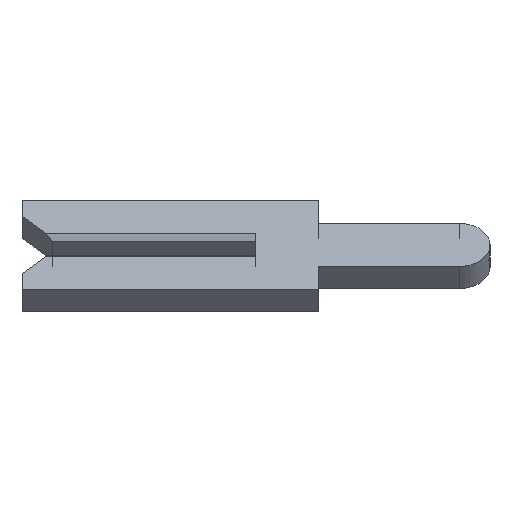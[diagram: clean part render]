
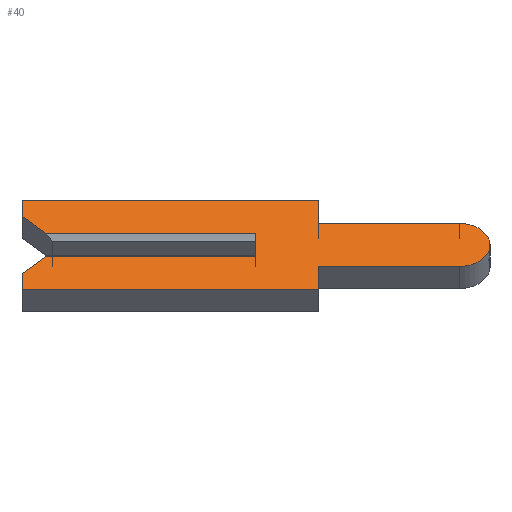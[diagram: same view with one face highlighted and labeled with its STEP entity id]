
A CAD part, left-side view. The second image highlights one B-rep face of the part: STEP entity #40.
In plain terms, the highlighted face is planar.
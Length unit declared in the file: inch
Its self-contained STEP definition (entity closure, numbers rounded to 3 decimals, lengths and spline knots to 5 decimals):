
#7 = CARTESIAN_POINT ( 'NONE',  ( -0.01, -0.1305, -0.0195 ) ) ;
#40 = ADVANCED_FACE ( 'NONE', ( #916 ), #999, .F. ) ;
#54 = CARTESIAN_POINT ( 'NONE',  ( -0.01, 0.15, -0.026 ) ) ;
#56 = ORIENTED_EDGE ( 'NONE', *, *, #1385, .F. ) ;
#73 = VERTEX_POINT ( 'NONE', #1260 ) ;
#75 = ORIENTED_EDGE ( 'NONE', *, *, #737, .T. ) ;
#84 = CARTESIAN_POINT ( 'NONE',  ( -0.01, 0.1305, 0.0065 ) ) ;
#95 = ORIENTED_EDGE ( 'NONE', *, *, #278, .F. ) ;
#117 = EDGE_CURVE ( 'NONE', #73, #673, #1563, .T. ) ;
#166 = VERTEX_POINT ( 'NONE', #751 ) ;
#167 = DIRECTION ( 'NONE',  ( 0., -1., 0. ) ) ;
#184 = VERTEX_POINT ( 'NONE', #244 ) ;
#197 = EDGE_CURVE ( 'NONE', #1098, #594, #1121, .T. ) ;
#206 = EDGE_CURVE ( 'NONE', #1483, #184, #1257, .T. ) ;
#219 = CARTESIAN_POINT ( 'NONE',  ( -0.01, -0.04, 0.0195 ) ) ;
#220 = VECTOR ( 'NONE', #1440, 39.37008 ) ;
#230 = ORIENTED_EDGE ( 'NONE', *, *, #1221, .F. ) ;
#234 = DIRECTION ( 'NONE',  ( 0., -1., 0. ) ) ;
#236 = LINE ( 'NONE', #606, #220 ) ;
#244 = CARTESIAN_POINT ( 'NONE',  ( -0.01, -0.04, -0.0195 ) ) ;
#247 = VECTOR ( 'NONE', #285, 39.37008 ) ;
#265 = EDGE_CURVE ( 'NONE', #673, #735, #1557, .T. ) ;
#269 = CARTESIAN_POINT ( 'NONE',  ( -0.01, 0.15, -0.026 ) ) ;
#278 = EDGE_CURVE ( 'NONE', #1012, #1098, #1266, .T. ) ;
#285 = DIRECTION ( 'NONE',  ( 0., -0.707, 0.707 ) ) ;
#288 = VERTEX_POINT ( 'NONE', #1540 ) ;
#307 = VECTOR ( 'NONE', #618, 39.37008 ) ;
#311 = CARTESIAN_POINT ( 'NONE',  ( -0.01, -0.04, 0.04 ) ) ;
#329 = CARTESIAN_POINT ( 'NONE',  ( -0.01, 0.134, -0.01 ) ) ;
#353 = CARTESIAN_POINT ( 'NONE',  ( -0.01, -0.1305, 0. ) ) ;
#406 = LINE ( 'NONE', #416, #780 ) ;
#416 = CARTESIAN_POINT ( 'NONE',  ( -0.01, 0.15, 0.01 ) ) ;
#423 = EDGE_CURVE ( 'NONE', #735, #1012, #580, .T. ) ;
#460 = LINE ( 'NONE', #1486, #898 ) ;
#465 = ORIENTED_EDGE ( 'NONE', *, *, #1082, .F. ) ;
#471 = DIRECTION ( 'NONE',  ( 1., 0., 0. ) ) ;
#481 = VECTOR ( 'NONE', #234, 39.37008 ) ;
#494 = DIRECTION ( 'NONE',  ( 0., 0., -1. ) ) ;
#540 = ORIENTED_EDGE ( 'NONE', *, *, #1000, .F. ) ;
#569 = AXIS2_PLACEMENT_3D ( 'NONE', #1506, #875, #494 ) ;
#580 = LINE ( 'NONE', #1154, #247 ) ;
#594 = VERTEX_POINT ( 'NONE', #672 ) ;
#598 = DIRECTION ( 'NONE',  ( 0., -1., 0. ) ) ;
#599 = ORIENTED_EDGE ( 'NONE', *, *, #423, .F. ) ;
#605 = LINE ( 'NONE', #940, #802 ) ;
#606 = CARTESIAN_POINT ( 'NONE',  ( -0.01, -0.04, -0.04 ) ) ;
#612 = CARTESIAN_POINT ( 'NONE',  ( -0.01, 0.15, 0.04 ) ) ;
#618 = DIRECTION ( 'NONE',  ( 0., 0., 1. ) ) ;
#635 = ORIENTED_EDGE ( 'NONE', *, *, #265, .F. ) ;
#672 = CARTESIAN_POINT ( 'NONE',  ( -0.01, 0., 0.01 ) ) ;
#673 = VERTEX_POINT ( 'NONE', #815 ) ;
#727 = ORIENTED_EDGE ( 'NONE', *, *, #206, .F. ) ;
#729 = DIRECTION ( 'NONE',  ( 0., 0., -1. ) ) ;
#735 = VERTEX_POINT ( 'NONE', #54 ) ;
#737 = EDGE_CURVE ( 'NONE', #288, #594, #406, .T. ) ;
#744 = VECTOR ( 'NONE', #956, 39.37008 ) ;
#751 = CARTESIAN_POINT ( 'NONE',  ( -0.01, 0.15, 0.04 ) ) ;
#754 = DIRECTION ( 'NONE',  ( 0., 1., 0. ) ) ;
#780 = VECTOR ( 'NONE', #167, 39.37008 ) ;
#802 = VECTOR ( 'NONE', #1096, 39.37008 ) ;
#815 = CARTESIAN_POINT ( 'NONE',  ( -0.01, 0.15, -0.04 ) ) ;
#832 = VERTEX_POINT ( 'NONE', #1432 ) ;
#867 = LINE ( 'NONE', #311, #1512 ) ;
#875 = DIRECTION ( 'NONE',  ( 1., 0., 0. ) ) ;
#886 = DIRECTION ( 'NONE',  ( 0., 1., 0. ) ) ;
#898 = VECTOR ( 'NONE', #598, 39.37008 ) ;
#913 = VECTOR ( 'NONE', #754, 39.37008 ) ;
#916 = FACE_OUTER_BOUND ( 'NONE', #1346, .T. ) ;
#940 = CARTESIAN_POINT ( 'NONE',  ( -0.01, 0.15, 0.026 ) ) ;
#945 = CARTESIAN_POINT ( 'NONE',  ( -0.01, 0.15, 0.026 ) ) ;
#956 = DIRECTION ( 'NONE',  ( 0., 0.707, 0.707 ) ) ;
#987 = CIRCLE ( 'NONE', #1458, 0.0195 ) ;
#990 = ORIENTED_EDGE ( 'NONE', *, *, #197, .F. ) ;
#991 = VECTOR ( 'NONE', #1518, 39.37008 ) ;
#999 = PLANE ( 'NONE',  #569 ) ;
#1000 = EDGE_CURVE ( 'NONE', #288, #1137, #1070, .T. ) ;
#1012 = VERTEX_POINT ( 'NONE', #329 ) ;
#1019 = DIRECTION ( 'NONE',  ( 0., -1., 0. ) ) ;
#1021 = ORIENTED_EDGE ( 'NONE', *, *, #1300, .F. ) ;
#1030 = EDGE_CURVE ( 'NONE', #1137, #166, #605, .T. ) ;
#1070 = LINE ( 'NONE', #84, #744 ) ;
#1082 = EDGE_CURVE ( 'NONE', #832, #1555, #867, .T. ) ;
#1096 = DIRECTION ( 'NONE',  ( 0., 0., 1. ) ) ;
#1098 = VERTEX_POINT ( 'NONE', #1451 ) ;
#1121 = LINE ( 'NONE', #1391, #307 ) ;
#1137 = VERTEX_POINT ( 'NONE', #945 ) ;
#1154 = CARTESIAN_POINT ( 'NONE',  ( -0.01, 0.1305, -0.0065 ) ) ;
#1168 = CARTESIAN_POINT ( 'NONE',  ( -0.01, -0.1305, -0.01 ) ) ;
#1214 = DIRECTION ( 'NONE',  ( 0., 0., -1. ) ) ;
#1221 = EDGE_CURVE ( 'NONE', #166, #832, #1491, .T. ) ;
#1227 = VECTOR ( 'NONE', #1019, 39.37008 ) ;
#1232 = CARTESIAN_POINT ( 'NONE',  ( -0.01, -0.1305, 0.0195 ) ) ;
#1233 = ORIENTED_EDGE ( 'NONE', *, *, #117, .F. ) ;
#1257 = LINE ( 'NONE', #1511, #913 ) ;
#1260 = CARTESIAN_POINT ( 'NONE',  ( -0.01, -0.04, -0.04 ) ) ;
#1266 = LINE ( 'NONE', #1168, #1227 ) ;
#1300 = EDGE_CURVE ( 'NONE', #1307, #1483, #987, .T. ) ;
#1307 = VERTEX_POINT ( 'NONE', #1232 ) ;
#1346 = EDGE_LOOP ( 'NONE', ( #75, #990, #95, #599, #635, #1233, #56, #727, #1021, #1417, #465, #230, #1538, #540 ) ) ;
#1361 = EDGE_CURVE ( 'NONE', #1555, #1307, #460, .T. ) ;
#1385 = EDGE_CURVE ( 'NONE', #184, #73, #236, .T. ) ;
#1391 = CARTESIAN_POINT ( 'NONE',  ( -0.01, 0., 0.0065 ) ) ;
#1417 = ORIENTED_EDGE ( 'NONE', *, *, #1361, .F. ) ;
#1432 = CARTESIAN_POINT ( 'NONE',  ( -0.01, -0.04, 0.04 ) ) ;
#1440 = DIRECTION ( 'NONE',  ( 0., 0., -1. ) ) ;
#1451 = CARTESIAN_POINT ( 'NONE',  ( -0.01, 0., -0.01 ) ) ;
#1458 = AXIS2_PLACEMENT_3D ( 'NONE', #353, #471, #729 ) ;
#1483 = VERTEX_POINT ( 'NONE', #7 ) ;
#1486 = CARTESIAN_POINT ( 'NONE',  ( -0.01, -0.04, 0.0195 ) ) ;
#1488 = CARTESIAN_POINT ( 'NONE',  ( -0.01, 0.15, -0.04 ) ) ;
#1491 = LINE ( 'NONE', #612, #481 ) ;
#1506 = CARTESIAN_POINT ( 'NONE',  ( -0.01, -0.1305, 0. ) ) ;
#1511 = CARTESIAN_POINT ( 'NONE',  ( -0.01, -0.04, -0.0195 ) ) ;
#1512 = VECTOR ( 'NONE', #1214, 39.37008 ) ;
#1518 = DIRECTION ( 'NONE',  ( 0., 0., 1. ) ) ;
#1526 = VECTOR ( 'NONE', #886, 39.37008 ) ;
#1538 = ORIENTED_EDGE ( 'NONE', *, *, #1030, .F. ) ;
#1540 = CARTESIAN_POINT ( 'NONE',  ( -0.01, 0.134, 0.01 ) ) ;
#1555 = VERTEX_POINT ( 'NONE', #219 ) ;
#1557 = LINE ( 'NONE', #269, #991 ) ;
#1563 = LINE ( 'NONE', #1488, #1526 ) ;
